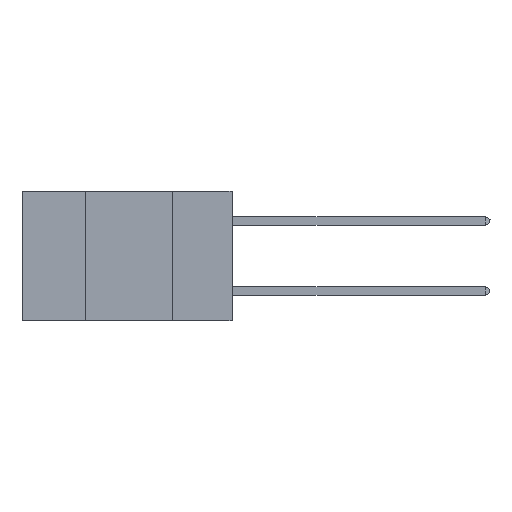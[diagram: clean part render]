
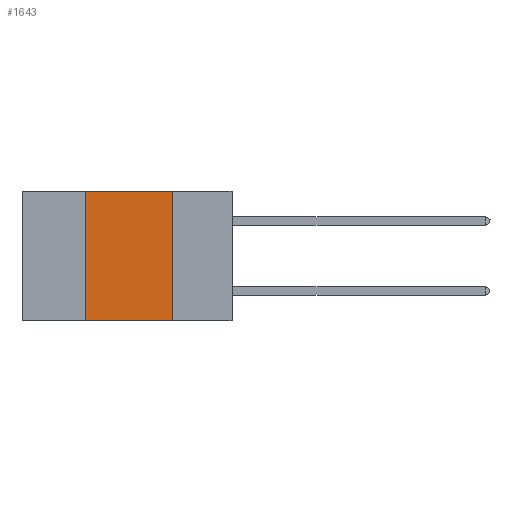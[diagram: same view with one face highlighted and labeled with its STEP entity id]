
A CAD part, left-side view. The second image highlights one B-rep face of the part: STEP entity #1643.
In plain terms, the highlighted planar face has unit normal (-1, 0, 0).
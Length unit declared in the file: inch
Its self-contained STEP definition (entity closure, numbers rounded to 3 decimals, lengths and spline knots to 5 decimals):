
#295 = VECTOR ( 'NONE', #3656, 39.37008 ) ;
#618 = ORIENTED_EDGE ( 'NONE', *, *, #21161, .F. ) ;
#1173 = VERTEX_POINT ( 'NONE', #7275 ) ;
#1235 = DIRECTION ( 'NONE',  ( 0., 0., -1. ) ) ;
#1253 = VERTEX_POINT ( 'NONE', #15826 ) ;
#1643 = ADVANCED_FACE ( 'NONE', ( #7369 ), #21671, .F. ) ;
#2204 = VECTOR ( 'NONE', #12541, 39.37008 ) ;
#2266 = AXIS2_PLACEMENT_3D ( 'NONE', #19792, #11243, #1235 ) ;
#2847 = ORIENTED_EDGE ( 'NONE', *, *, #4348, .F. ) ;
#3656 = DIRECTION ( 'NONE',  ( 0., 0., 1. ) ) ;
#4348 = EDGE_CURVE ( 'NONE', #19589, #1253, #18691, .T. ) ;
#4392 = LINE ( 'NONE', #18819, #2204 ) ;
#4760 = EDGE_LOOP ( 'NONE', ( #2847, #618, #15798, #6485 ) ) ;
#4899 = VECTOR ( 'NONE', #18560, 39.37008 ) ;
#6485 = ORIENTED_EDGE ( 'NONE', *, *, #12289, .T. ) ;
#7275 = CARTESIAN_POINT ( 'NONE',  ( 0., 0.42, -0.37 ) ) ;
#7369 = FACE_OUTER_BOUND ( 'NONE', #4760, .T. ) ;
#8238 = CARTESIAN_POINT ( 'NONE',  ( 0., 0.6, 0. ) ) ;
#8507 = LINE ( 'NONE', #8238, #8737 ) ;
#8737 = VECTOR ( 'NONE', #16394, 39.37008 ) ;
#9631 = EDGE_CURVE ( 'NONE', #1173, #18050, #21963, .T. ) ;
#11243 = DIRECTION ( 'NONE',  ( 1., 0., 0. ) ) ;
#12289 = EDGE_CURVE ( 'NONE', #1173, #1253, #4392, .T. ) ;
#12541 = DIRECTION ( 'NONE',  ( 0., -1., 0. ) ) ;
#15798 = ORIENTED_EDGE ( 'NONE', *, *, #9631, .F. ) ;
#15826 = CARTESIAN_POINT ( 'NONE',  ( 0., 0.17, -0.37 ) ) ;
#16218 = CARTESIAN_POINT ( 'NONE',  ( 0., 0.42, 0. ) ) ;
#16394 = DIRECTION ( 'NONE',  ( 0., -1., 0. ) ) ;
#16551 = CARTESIAN_POINT ( 'NONE',  ( 0., 0.17, 0. ) ) ;
#16708 = CARTESIAN_POINT ( 'NONE',  ( 0., 0.42, 0. ) ) ;
#18050 = VERTEX_POINT ( 'NONE', #16708 ) ;
#18560 = DIRECTION ( 'NONE',  ( 0., 0., -1. ) ) ;
#18691 = LINE ( 'NONE', #16551, #4899 ) ;
#18819 = CARTESIAN_POINT ( 'NONE',  ( 0., 0.6, -0.37 ) ) ;
#19589 = VERTEX_POINT ( 'NONE', #25436 ) ;
#19792 = CARTESIAN_POINT ( 'NONE',  ( 0., 0.6, 0. ) ) ;
#21161 = EDGE_CURVE ( 'NONE', #18050, #19589, #8507, .T. ) ;
#21671 = PLANE ( 'NONE',  #2266 ) ;
#21963 = LINE ( 'NONE', #16218, #295 ) ;
#25436 = CARTESIAN_POINT ( 'NONE',  ( 0., 0.17, 0. ) ) ;
